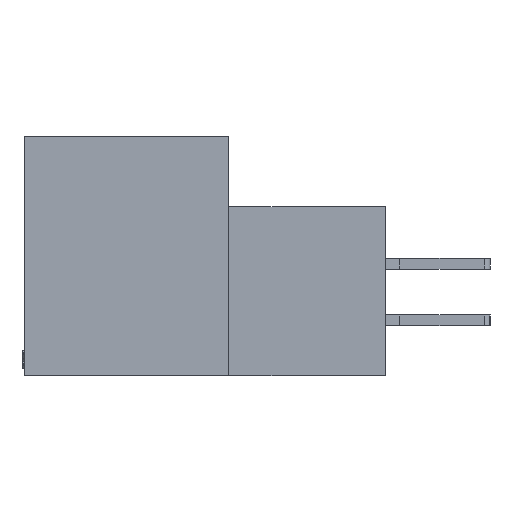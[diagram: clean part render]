
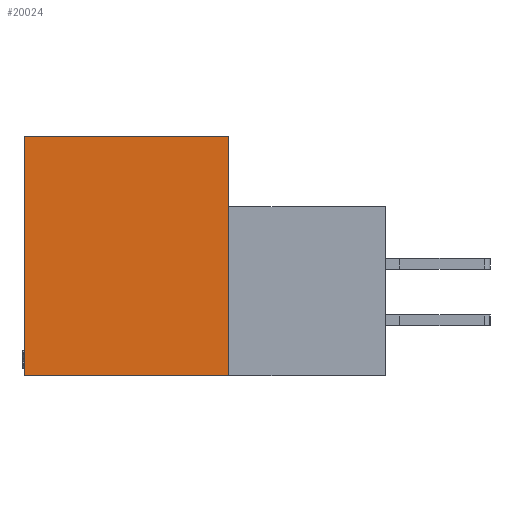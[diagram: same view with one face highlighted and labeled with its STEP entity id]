
A CAD part, left-side view. The second image highlights one B-rep face of the part: STEP entity #20024.
In plain terms, the highlighted planar face has unit normal (-1, 0, 0).
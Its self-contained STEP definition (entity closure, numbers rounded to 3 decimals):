
#7 = CARTESIAN_POINT ( 'NONE',  ( 0., 0., 0. ) ) ;
#64 = DIRECTION ( 'NONE',  ( 0., 1., 0. ) ) ;
#1955 = ORIENTED_EDGE ( 'NONE', *, *, #9609, .F. ) ;
#1976 = VECTOR ( 'NONE', #3358, 1000. ) ;
#3358 = DIRECTION ( 'NONE',  ( 0., 0., -1. ) ) ;
#4085 = CARTESIAN_POINT ( 'NONE',  ( 0., 11.506, 0. ) ) ;
#4378 = DIRECTION ( 'NONE',  ( 0., -1., 0. ) ) ;
#5440 = LINE ( 'NONE', #20850, #25262 ) ;
#6396 = VECTOR ( 'NONE', #4378, 1000. ) ;
#6970 = EDGE_CURVE ( 'NONE', #15232, #20756, #15380, .T. ) ;
#7298 = DIRECTION ( 'NONE',  ( 0., 0., 1. ) ) ;
#7881 = CARTESIAN_POINT ( 'NONE',  ( 0., 0., 0. ) ) ;
#8065 = EDGE_CURVE ( 'NONE', #20756, #22879, #5440, .T. ) ;
#8338 = EDGE_LOOP ( 'NONE', ( #24549, #19118, #1955, #28512 ) ) ;
#9609 = EDGE_CURVE ( 'NONE', #22879, #22078, #28705, .T. ) ;
#10525 = FACE_OUTER_BOUND ( 'NONE', #8338, .T. ) ;
#11765 = CARTESIAN_POINT ( 'NONE',  ( 0., 11.506, 0. ) ) ;
#12633 = AXIS2_PLACEMENT_3D ( 'NONE', #7, #29189, #22659 ) ;
#13210 = CARTESIAN_POINT ( 'NONE',  ( 0., -8.814, -13.487 ) ) ;
#15232 = VERTEX_POINT ( 'NONE', #24468 ) ;
#15380 = LINE ( 'NONE', #13210, #26379 ) ;
#15584 = EDGE_CURVE ( 'NONE', #22078, #15232, #26035, .T. ) ;
#19118 = ORIENTED_EDGE ( 'NONE', *, *, #15584, .F. ) ;
#20024 = ADVANCED_FACE ( 'NONE', ( #10525 ), #20161, .F. ) ;
#20161 = PLANE ( 'NONE',  #12633 ) ;
#20756 = VERTEX_POINT ( 'NONE', #25031 ) ;
#20850 = CARTESIAN_POINT ( 'NONE',  ( 0., 11.506, -13.487 ) ) ;
#22078 = VERTEX_POINT ( 'NONE', #24285 ) ;
#22659 = DIRECTION ( 'NONE',  ( 0., 0., -1. ) ) ;
#22879 = VERTEX_POINT ( 'NONE', #11765 ) ;
#24285 = CARTESIAN_POINT ( 'NONE',  ( 0., 0., 0. ) ) ;
#24468 = CARTESIAN_POINT ( 'NONE',  ( 0., 0., -13.487 ) ) ;
#24549 = ORIENTED_EDGE ( 'NONE', *, *, #6970, .F. ) ;
#25031 = CARTESIAN_POINT ( 'NONE',  ( 0., 11.506, -13.487 ) ) ;
#25262 = VECTOR ( 'NONE', #7298, 1000. ) ;
#26035 = LINE ( 'NONE', #7881, #1976 ) ;
#26379 = VECTOR ( 'NONE', #64, 1000. ) ;
#28512 = ORIENTED_EDGE ( 'NONE', *, *, #8065, .F. ) ;
#28705 = LINE ( 'NONE', #4085, #6396 ) ;
#29189 = DIRECTION ( 'NONE',  ( 1., 0., 0. ) ) ;
